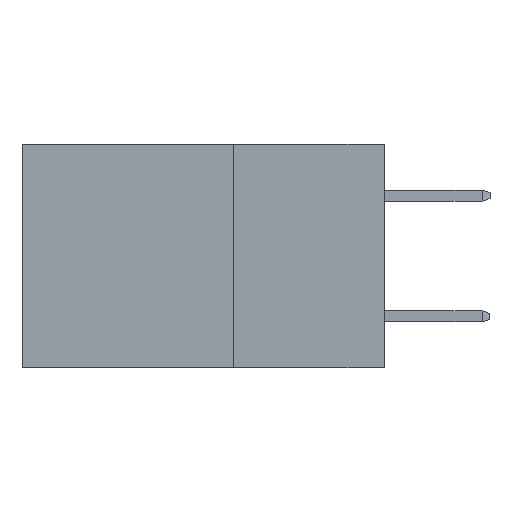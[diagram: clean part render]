
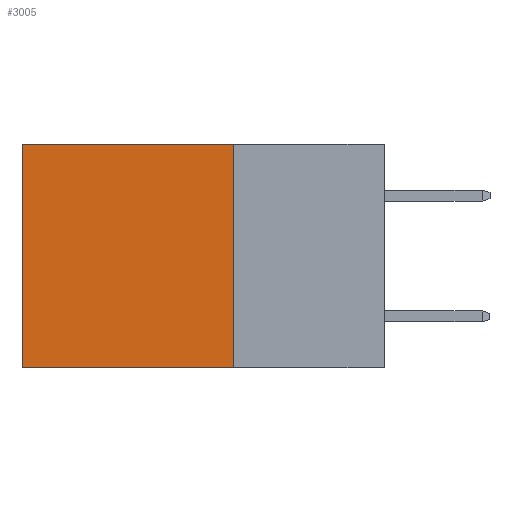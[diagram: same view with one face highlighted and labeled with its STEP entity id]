
A CAD part, left-side view. The second image highlights one B-rep face of the part: STEP entity #3005.
In plain terms, the highlighted planar face has unit normal (-1, 0, 0).
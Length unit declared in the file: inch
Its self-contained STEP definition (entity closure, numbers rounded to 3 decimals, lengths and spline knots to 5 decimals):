
#404 = DIRECTION ( 'NONE',  ( 0., 0., -1. ) ) ;
#804 = CARTESIAN_POINT ( 'NONE',  ( 0.298, 0.25, -0.37 ) ) ;
#1449 = LINE ( 'NONE', #8760, #5747 ) ;
#1457 = LINE ( 'NONE', #804, #6003 ) ;
#2134 = ORIENTED_EDGE ( 'NONE', *, *, #10323, .T. ) ;
#2530 = CARTESIAN_POINT ( 'NONE',  ( 0.298, 0.6, -0.37 ) ) ;
#2549 = ORIENTED_EDGE ( 'NONE', *, *, #5712, .F. ) ;
#2599 = ORIENTED_EDGE ( 'NONE', *, *, #5944, .F. ) ;
#2779 = DIRECTION ( 'NONE',  ( 0., 0., -1. ) ) ;
#2872 = ORIENTED_EDGE ( 'NONE', *, *, #6590, .T. ) ;
#3005 = ADVANCED_FACE ( 'NONE', ( #4266 ), #7812, .F. ) ;
#3134 = VERTEX_POINT ( 'NONE', #2530 ) ;
#3200 = EDGE_LOOP ( 'NONE', ( #2134, #2549, #2599, #2872 ) ) ;
#3307 = CARTESIAN_POINT ( 'NONE',  ( 0.298, 0.6, 0. ) ) ;
#3995 = AXIS2_PLACEMENT_3D ( 'NONE', #6096, #8349, #2779 ) ;
#4080 = CARTESIAN_POINT ( 'NONE',  ( 0.298, 0.25, 0. ) ) ;
#4266 = FACE_OUTER_BOUND ( 'NONE', #3200, .T. ) ;
#4679 = CARTESIAN_POINT ( 'NONE',  ( 0.298, 0.25, 0. ) ) ;
#5637 = DIRECTION ( 'NONE',  ( 0., 0., -1. ) ) ;
#5712 = EDGE_CURVE ( 'NONE', #8900, #3134, #1457, .T. ) ;
#5747 = VECTOR ( 'NONE', #5637, 39.37008 ) ;
#5944 = EDGE_CURVE ( 'NONE', #7494, #8900, #6215, .T. ) ;
#6003 = VECTOR ( 'NONE', #9076, 39.37008 ) ;
#6096 = CARTESIAN_POINT ( 'NONE',  ( 0.298, 0.25, 0. ) ) ;
#6215 = LINE ( 'NONE', #10276, #10130 ) ;
#6590 = EDGE_CURVE ( 'NONE', #7494, #8212, #7666, .T. ) ;
#7494 = VERTEX_POINT ( 'NONE', #4080 ) ;
#7666 = LINE ( 'NONE', #4679, #9513 ) ;
#7812 = PLANE ( 'NONE',  #3995 ) ;
#7865 = DIRECTION ( 'NONE',  ( 0., 1., 0. ) ) ;
#8212 = VERTEX_POINT ( 'NONE', #3307 ) ;
#8349 = DIRECTION ( 'NONE',  ( 1., 0., 0. ) ) ;
#8760 = CARTESIAN_POINT ( 'NONE',  ( 0.298, 0.6, 0. ) ) ;
#8900 = VERTEX_POINT ( 'NONE', #8994 ) ;
#8994 = CARTESIAN_POINT ( 'NONE',  ( 0.298, 0.25, -0.37 ) ) ;
#9076 = DIRECTION ( 'NONE',  ( 0., 1., 0. ) ) ;
#9513 = VECTOR ( 'NONE', #7865, 39.37008 ) ;
#10130 = VECTOR ( 'NONE', #404, 39.37008 ) ;
#10276 = CARTESIAN_POINT ( 'NONE',  ( 0.298, 0.25, 0. ) ) ;
#10323 = EDGE_CURVE ( 'NONE', #8212, #3134, #1449, .T. ) ;
